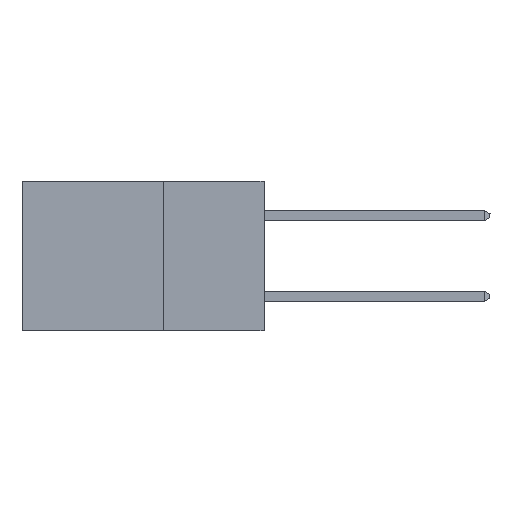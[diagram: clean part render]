
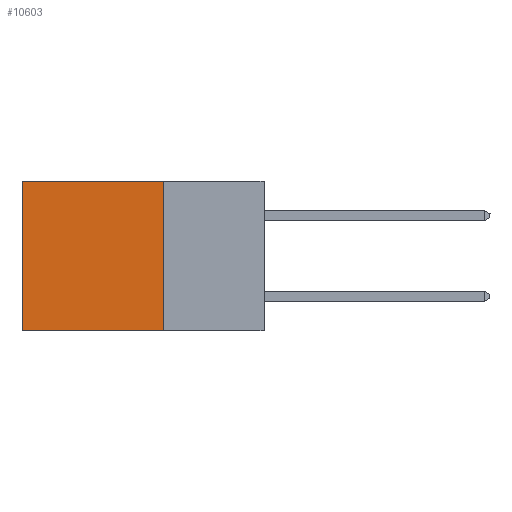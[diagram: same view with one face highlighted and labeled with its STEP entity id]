
A CAD part, left-side view. The second image highlights one B-rep face of the part: STEP entity #10603.
In plain terms, the highlighted planar face has unit normal (-1, 0, 0).
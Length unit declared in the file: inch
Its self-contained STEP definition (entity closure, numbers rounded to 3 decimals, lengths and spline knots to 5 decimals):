
#354 = DIRECTION ( 'NONE',  ( 0., 0., -1. ) ) ;
#1389 = LINE ( 'NONE', #6956, #13455 ) ;
#1799 = ORIENTED_EDGE ( 'NONE', *, *, #33060, .F. ) ;
#2648 = VECTOR ( 'NONE', #354, 39.37008 ) ;
#5612 = CARTESIAN_POINT ( 'NONE',  ( 0.298, 0.6, -0.37 ) ) ;
#6180 = CARTESIAN_POINT ( 'NONE',  ( 0.298, 0.25, 0. ) ) ;
#6846 = VERTEX_POINT ( 'NONE', #5612 ) ;
#6956 = CARTESIAN_POINT ( 'NONE',  ( 0.298, 0.25, 0. ) ) ;
#8205 = VERTEX_POINT ( 'NONE', #27211 ) ;
#8794 = PLANE ( 'NONE',  #10539 ) ;
#9214 = ORIENTED_EDGE ( 'NONE', *, *, #15055, .T. ) ;
#9305 = VECTOR ( 'NONE', #31576, 39.37008 ) ;
#9562 = DIRECTION ( 'NONE',  ( 0., 1., 0. ) ) ;
#10416 = VERTEX_POINT ( 'NONE', #10617 ) ;
#10539 = AXIS2_PLACEMENT_3D ( 'NONE', #6180, #11388, #29243 ) ;
#10603 = ADVANCED_FACE ( 'NONE', ( #13254 ), #8794, .F. ) ;
#10617 = CARTESIAN_POINT ( 'NONE',  ( 0.298, 0.6, 0. ) ) ;
#11136 = CARTESIAN_POINT ( 'NONE',  ( 0.298, 0.25, 0. ) ) ;
#11388 = DIRECTION ( 'NONE',  ( 1., 0., 0. ) ) ;
#13254 = FACE_OUTER_BOUND ( 'NONE', #18527, .T. ) ;
#13455 = VECTOR ( 'NONE', #9562, 39.37008 ) ;
#13493 = ORIENTED_EDGE ( 'NONE', *, *, #29155, .F. ) ;
#14884 = CARTESIAN_POINT ( 'NONE',  ( 0.298, 0.25, -0.37 ) ) ;
#15055 = EDGE_CURVE ( 'NONE', #8205, #10416, #1389, .T. ) ;
#16298 = LINE ( 'NONE', #31298, #2648 ) ;
#17474 = DIRECTION ( 'NONE',  ( 0., 1., 0. ) ) ;
#18527 = EDGE_LOOP ( 'NONE', ( #23570, #13493, #1799, #9214 ) ) ;
#20756 = VECTOR ( 'NONE', #17474, 39.37008 ) ;
#21391 = EDGE_CURVE ( 'NONE', #10416, #6846, #16298, .T. ) ;
#23570 = ORIENTED_EDGE ( 'NONE', *, *, #21391, .T. ) ;
#24486 = LINE ( 'NONE', #11136, #9305 ) ;
#25771 = VERTEX_POINT ( 'NONE', #25843 ) ;
#25843 = CARTESIAN_POINT ( 'NONE',  ( 0.298, 0.25, -0.37 ) ) ;
#27211 = CARTESIAN_POINT ( 'NONE',  ( 0.298, 0.25, 0. ) ) ;
#27491 = LINE ( 'NONE', #14884, #20756 ) ;
#29155 = EDGE_CURVE ( 'NONE', #25771, #6846, #27491, .T. ) ;
#29243 = DIRECTION ( 'NONE',  ( 0., 0., -1. ) ) ;
#31298 = CARTESIAN_POINT ( 'NONE',  ( 0.298, 0.6, 0. ) ) ;
#31576 = DIRECTION ( 'NONE',  ( 0., 0., -1. ) ) ;
#33060 = EDGE_CURVE ( 'NONE', #8205, #25771, #24486, .T. ) ;
